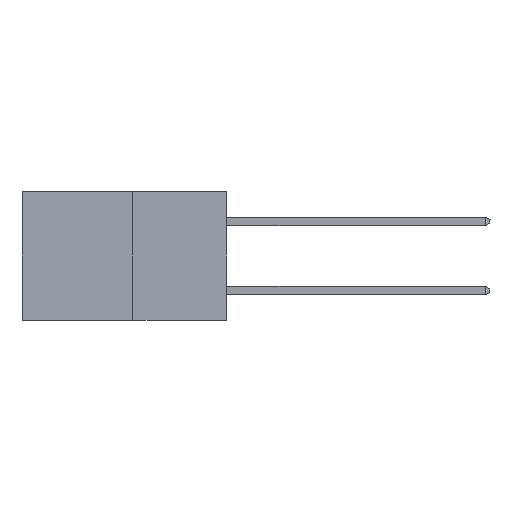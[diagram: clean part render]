
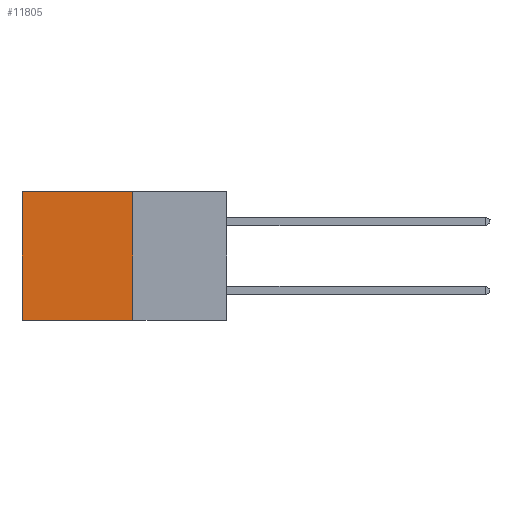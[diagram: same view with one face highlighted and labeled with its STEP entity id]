
A CAD part, left-side view. The second image highlights one B-rep face of the part: STEP entity #11805.
In plain terms, the highlighted planar face has unit normal (-1, 0, 0).
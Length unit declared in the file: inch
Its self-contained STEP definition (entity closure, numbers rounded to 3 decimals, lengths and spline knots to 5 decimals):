
#162 = EDGE_CURVE ( 'NONE', #5898, #7571, #11053, .T. ) ;
#1221 = VECTOR ( 'NONE', #11923, 39.37008 ) ;
#1673 = DIRECTION ( 'NONE',  ( 0., 0., -1. ) ) ;
#1703 = CARTESIAN_POINT ( 'NONE',  ( 0.277, 0.59, -0.37 ) ) ;
#2008 = CARTESIAN_POINT ( 'NONE',  ( 0.277, 0.27, -0.37 ) ) ;
#2180 = DIRECTION ( 'NONE',  ( 0., 0., -1. ) ) ;
#3057 = VECTOR ( 'NONE', #1673, 39.37008 ) ;
#3061 = AXIS2_PLACEMENT_3D ( 'NONE', #13412, #14112, #14098 ) ;
#3927 = ORIENTED_EDGE ( 'NONE', *, *, #11415, .T. ) ;
#5186 = CARTESIAN_POINT ( 'NONE',  ( 0.277, 0.27, 0. ) ) ;
#5687 = CARTESIAN_POINT ( 'NONE',  ( 0.277, 0.27, 0. ) ) ;
#5898 = VERTEX_POINT ( 'NONE', #5186 ) ;
#6453 = EDGE_CURVE ( 'NONE', #5898, #9039, #12591, .T. ) ;
#6606 = VERTEX_POINT ( 'NONE', #7563 ) ;
#6659 = EDGE_CURVE ( 'NONE', #9039, #6606, #9319, .T. ) ;
#6686 = LINE ( 'NONE', #1703, #3057 ) ;
#7563 = CARTESIAN_POINT ( 'NONE',  ( 0.277, 0.59, -0.37 ) ) ;
#7571 = VERTEX_POINT ( 'NONE', #8256 ) ;
#7602 = FACE_OUTER_BOUND ( 'NONE', #19561, .T. ) ;
#8256 = CARTESIAN_POINT ( 'NONE',  ( 0.277, 0.59, 0. ) ) ;
#8656 = VECTOR ( 'NONE', #2180, 39.37008 ) ;
#9039 = VERTEX_POINT ( 'NONE', #14356 ) ;
#9319 = LINE ( 'NONE', #11304, #1221 ) ;
#9917 = DIRECTION ( 'NONE',  ( 0., 1., 0. ) ) ;
#9920 = ORIENTED_EDGE ( 'NONE', *, *, #162, .T. ) ;
#11053 = LINE ( 'NONE', #5687, #18650 ) ;
#11304 = CARTESIAN_POINT ( 'NONE',  ( 0.277, 0.27, -0.37 ) ) ;
#11415 = EDGE_CURVE ( 'NONE', #7571, #6606, #6686, .T. ) ;
#11805 = ADVANCED_FACE ( 'NONE', ( #7602 ), #14436, .F. ) ;
#11923 = DIRECTION ( 'NONE',  ( 0., 1., 0. ) ) ;
#12062 = ORIENTED_EDGE ( 'NONE', *, *, #6659, .F. ) ;
#12591 = LINE ( 'NONE', #2008, #8656 ) ;
#13412 = CARTESIAN_POINT ( 'NONE',  ( 0.277, 0.27, -0.37 ) ) ;
#14098 = DIRECTION ( 'NONE',  ( 0., 0., -1. ) ) ;
#14112 = DIRECTION ( 'NONE',  ( 1., 0., 0. ) ) ;
#14356 = CARTESIAN_POINT ( 'NONE',  ( 0.277, 0.27, -0.37 ) ) ;
#14436 = PLANE ( 'NONE',  #3061 ) ;
#18650 = VECTOR ( 'NONE', #9917, 39.37008 ) ;
#19023 = ORIENTED_EDGE ( 'NONE', *, *, #6453, .F. ) ;
#19561 = EDGE_LOOP ( 'NONE', ( #3927, #12062, #19023, #9920 ) ) ;
